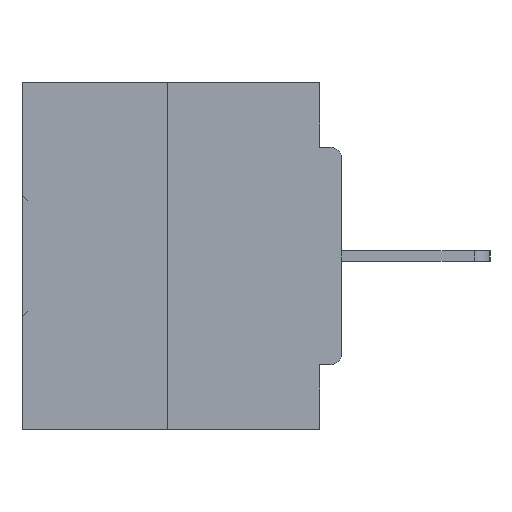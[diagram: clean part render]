
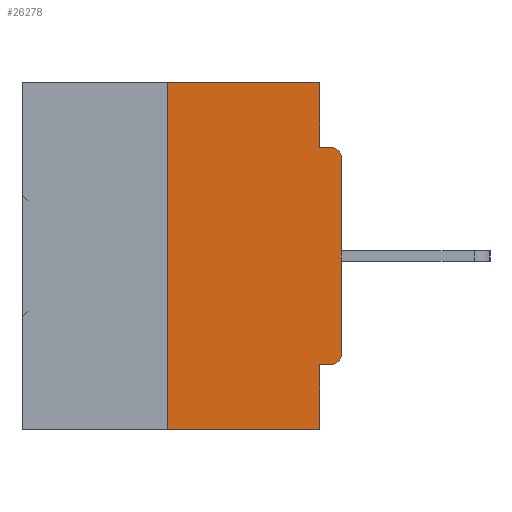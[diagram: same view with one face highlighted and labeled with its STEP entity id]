
A CAD part, left-side view. The second image highlights one B-rep face of the part: STEP entity #26278.
In plain terms, the highlighted planar face has unit normal (-1, 0, 0).
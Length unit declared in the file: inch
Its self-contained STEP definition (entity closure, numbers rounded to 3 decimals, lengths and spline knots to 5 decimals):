
#98 = VECTOR ( 'NONE', #20428, 39.37008 ) ;
#291 = AXIS2_PLACEMENT_3D ( 'NONE', #35732, #17447, #38798 ) ;
#804 = ORIENTED_EDGE ( 'NONE', *, *, #10148, .F. ) ;
#1893 = LINE ( 'NONE', #34384, #25683 ) ;
#1973 = EDGE_CURVE ( 'NONE', #18595, #18112, #3432, .T. ) ;
#3432 = LINE ( 'NONE', #19397, #35231 ) ;
#5266 = CARTESIAN_POINT ( 'NONE',  ( 0., 0., -0.3915 ) ) ;
#6720 = ORIENTED_EDGE ( 'NONE', *, *, #19454, .F. ) ;
#6859 = VERTEX_POINT ( 'NONE', #16995 ) ;
#7281 = DIRECTION ( 'NONE',  ( 0., 1., 0. ) ) ;
#8906 = DIRECTION ( 'NONE',  ( 0., -1., 0. ) ) ;
#9628 = DIRECTION ( 'NONE',  ( 0., 0., -1. ) ) ;
#10112 = CARTESIAN_POINT ( 'NONE',  ( 0., 0.031, -0.5 ) ) ;
#10148 = EDGE_CURVE ( 'NONE', #15342, #36278, #16684, .T. ) ;
#11263 = EDGE_LOOP ( 'NONE', ( #804, #26505, #12075, #36493, #6720, #31252, #16914, #33144, #27009, #36036 ) ) ;
#11644 = CARTESIAN_POINT ( 'NONE',  ( 0., 0.031, -0.0935 ) ) ;
#11686 = LINE ( 'NONE', #22399, #26132 ) ;
#12075 = ORIENTED_EDGE ( 'NONE', *, *, #15296, .T. ) ;
#12536 = EDGE_CURVE ( 'NONE', #36278, #36920, #17915, .T. ) ;
#12918 = LINE ( 'NONE', #18001, #37317 ) ;
#13521 = VECTOR ( 'NONE', #7281, 39.37008 ) ;
#13730 = CARTESIAN_POINT ( 'NONE',  ( 0., 0.015, -0.1085 ) ) ;
#15296 = EDGE_CURVE ( 'NONE', #35482, #18112, #35417, .T. ) ;
#15342 = VERTEX_POINT ( 'NONE', #39715 ) ;
#16378 = VERTEX_POINT ( 'NONE', #29807 ) ;
#16684 = LINE ( 'NONE', #17351, #98 ) ;
#16831 = DIRECTION ( 'NONE',  ( 0., 0., -1. ) ) ;
#16914 = ORIENTED_EDGE ( 'NONE', *, *, #24458, .T. ) ;
#16995 = CARTESIAN_POINT ( 'NONE',  ( 0., 0.015, -0.4065 ) ) ;
#17351 = CARTESIAN_POINT ( 'NONE',  ( 0., 0.46, 0. ) ) ;
#17447 = DIRECTION ( 'NONE',  ( -1., 0., 0. ) ) ;
#17915 = LINE ( 'NONE', #34028, #33176 ) ;
#18001 = CARTESIAN_POINT ( 'NONE',  ( 0., 0., 0. ) ) ;
#18011 = VERTEX_POINT ( 'NONE', #37177 ) ;
#18046 = EDGE_CURVE ( 'NONE', #35482, #15342, #1893, .T. ) ;
#18112 = VERTEX_POINT ( 'NONE', #10112 ) ;
#18595 = VERTEX_POINT ( 'NONE', #36877 ) ;
#19293 = DIRECTION ( 'NONE',  ( 0., -1., 0. ) ) ;
#19397 = CARTESIAN_POINT ( 'NONE',  ( 0., 0.031, -0.5 ) ) ;
#19454 = EDGE_CURVE ( 'NONE', #6859, #18595, #36964, .T. ) ;
#20428 = DIRECTION ( 'NONE',  ( 0., -1., 0. ) ) ;
#20792 = VERTEX_POINT ( 'NONE', #5266 ) ;
#21040 = DIRECTION ( 'NONE',  ( 0., 0., -1. ) ) ;
#21214 = CARTESIAN_POINT ( 'NONE',  ( 0., 0.46, -0.5 ) ) ;
#22141 = DIRECTION ( 'NONE',  ( 0., 0., 1. ) ) ;
#22399 = CARTESIAN_POINT ( 'NONE',  ( 0., 0., -0.0935 ) ) ;
#22410 = EDGE_CURVE ( 'NONE', #18011, #16378, #25115, .T. ) ;
#23564 = FACE_OUTER_BOUND ( 'NONE', #11263, .T. ) ;
#24201 = DIRECTION ( 'NONE',  ( 0., 0., 1. ) ) ;
#24458 = EDGE_CURVE ( 'NONE', #20792, #18011, #12918, .T. ) ;
#25115 = CIRCLE ( 'NONE', #32941, 0.015 ) ;
#25683 = VECTOR ( 'NONE', #22141, 39.37008 ) ;
#25779 = CARTESIAN_POINT ( 'NONE',  ( 0., 0., -0.4065 ) ) ;
#26132 = VECTOR ( 'NONE', #19293, 39.37008 ) ;
#26278 = ADVANCED_FACE ( 'NONE', ( #23564 ), #39160, .F. ) ;
#26394 = VECTOR ( 'NONE', #8906, 39.37008 ) ;
#26505 = ORIENTED_EDGE ( 'NONE', *, *, #18046, .F. ) ;
#27009 = ORIENTED_EDGE ( 'NONE', *, *, #30203, .F. ) ;
#27381 = EDGE_CURVE ( 'NONE', #6859, #20792, #29176, .T. ) ;
#29176 = CIRCLE ( 'NONE', #291, 0.015 ) ;
#29807 = CARTESIAN_POINT ( 'NONE',  ( 0., 0.015, -0.0935 ) ) ;
#30108 = CARTESIAN_POINT ( 'NONE',  ( 0., 0.46, 0. ) ) ;
#30203 = EDGE_CURVE ( 'NONE', #36920, #16378, #11686, .T. ) ;
#31252 = ORIENTED_EDGE ( 'NONE', *, *, #27381, .T. ) ;
#32941 = AXIS2_PLACEMENT_3D ( 'NONE', #13730, #35121, #16831 ) ;
#32980 = CARTESIAN_POINT ( 'NONE',  ( 0., 0.031, 0. ) ) ;
#33144 = ORIENTED_EDGE ( 'NONE', *, *, #22410, .T. ) ;
#33176 = VECTOR ( 'NONE', #9628, 39.37008 ) ;
#34028 = CARTESIAN_POINT ( 'NONE',  ( 0., 0.031, 0. ) ) ;
#34384 = CARTESIAN_POINT ( 'NONE',  ( 0., 0.25, 0. ) ) ;
#34393 = CARTESIAN_POINT ( 'NONE',  ( 0., 0.25, -0.5 ) ) ;
#35121 = DIRECTION ( 'NONE',  ( -1., 0., 0. ) ) ;
#35136 = AXIS2_PLACEMENT_3D ( 'NONE', #30108, #39291, #21040 ) ;
#35231 = VECTOR ( 'NONE', #37394, 39.37008 ) ;
#35417 = LINE ( 'NONE', #21214, #26394 ) ;
#35482 = VERTEX_POINT ( 'NONE', #34393 ) ;
#35732 = CARTESIAN_POINT ( 'NONE',  ( 0., 0.015, -0.3915 ) ) ;
#36036 = ORIENTED_EDGE ( 'NONE', *, *, #12536, .F. ) ;
#36278 = VERTEX_POINT ( 'NONE', #32980 ) ;
#36493 = ORIENTED_EDGE ( 'NONE', *, *, #1973, .F. ) ;
#36877 = CARTESIAN_POINT ( 'NONE',  ( 0., 0.031, -0.4065 ) ) ;
#36920 = VERTEX_POINT ( 'NONE', #11644 ) ;
#36964 = LINE ( 'NONE', #25779, #13521 ) ;
#37177 = CARTESIAN_POINT ( 'NONE',  ( 0., 0., -0.1085 ) ) ;
#37317 = VECTOR ( 'NONE', #24201, 39.37008 ) ;
#37394 = DIRECTION ( 'NONE',  ( 0., 0., -1. ) ) ;
#38798 = DIRECTION ( 'NONE',  ( 0., 0., -1. ) ) ;
#39160 = PLANE ( 'NONE',  #35136 ) ;
#39291 = DIRECTION ( 'NONE',  ( 1., 0., 0. ) ) ;
#39715 = CARTESIAN_POINT ( 'NONE',  ( 0., 0.25, 0. ) ) ;
